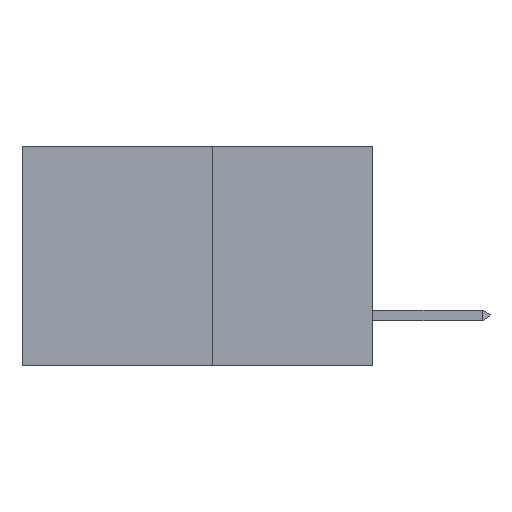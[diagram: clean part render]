
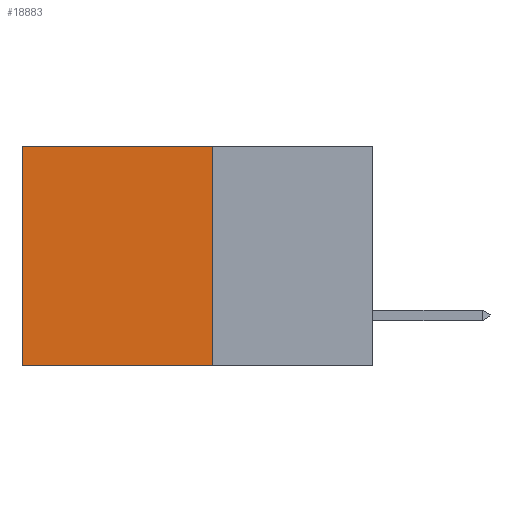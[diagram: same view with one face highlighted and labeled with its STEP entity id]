
A CAD part, left-side view. The second image highlights one B-rep face of the part: STEP entity #18883.
In plain terms, the highlighted planar face has unit normal (-1, 0, 0).
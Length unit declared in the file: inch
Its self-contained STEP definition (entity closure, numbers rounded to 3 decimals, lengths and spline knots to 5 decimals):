
#272 = LINE ( 'NONE', #681, #4980 ) ;
#427 = EDGE_CURVE ( 'NONE', #2098, #13107, #19022, .T. ) ;
#681 = CARTESIAN_POINT ( 'NONE',  ( 0.277, 0.27, -0.37 ) ) ;
#1015 = EDGE_CURVE ( 'NONE', #2098, #16600, #272, .T. ) ;
#1084 = VERTEX_POINT ( 'NONE', #19556 ) ;
#1745 = ORIENTED_EDGE ( 'NONE', *, *, #427, .T. ) ;
#1899 = CARTESIAN_POINT ( 'NONE',  ( 0.277, 0.27, 0. ) ) ;
#1974 = PLANE ( 'NONE',  #19280 ) ;
#2070 = DIRECTION ( 'NONE',  ( 1., 0., 0. ) ) ;
#2098 = VERTEX_POINT ( 'NONE', #1899 ) ;
#4743 = CARTESIAN_POINT ( 'NONE',  ( 0.277, 0.59, -0.37 ) ) ;
#4980 = VECTOR ( 'NONE', #21297, 39.37008 ) ;
#5964 = VECTOR ( 'NONE', #14572, 39.37008 ) ;
#6380 = CARTESIAN_POINT ( 'NONE',  ( 0.277, 0.27, -0.37 ) ) ;
#6897 = CARTESIAN_POINT ( 'NONE',  ( 0.277, 0.27, -0.37 ) ) ;
#6919 = DIRECTION ( 'NONE',  ( 0., 1., 0. ) ) ;
#7645 = LINE ( 'NONE', #6897, #13396 ) ;
#7882 = EDGE_CURVE ( 'NONE', #16600, #1084, #7645, .T. ) ;
#8899 = ORIENTED_EDGE ( 'NONE', *, *, #1015, .F. ) ;
#11194 = LINE ( 'NONE', #4743, #5964 ) ;
#11856 = EDGE_LOOP ( 'NONE', ( #18577, #19466, #8899, #1745 ) ) ;
#12308 = CARTESIAN_POINT ( 'NONE',  ( 0.277, 0.27, 0. ) ) ;
#13107 = VERTEX_POINT ( 'NONE', #17958 ) ;
#13396 = VECTOR ( 'NONE', #6919, 39.37008 ) ;
#13829 = CARTESIAN_POINT ( 'NONE',  ( 0.277, 0.27, -0.37 ) ) ;
#14572 = DIRECTION ( 'NONE',  ( 0., 0., -1. ) ) ;
#15781 = DIRECTION ( 'NONE',  ( 0., 0., -1. ) ) ;
#16600 = VERTEX_POINT ( 'NONE', #6380 ) ;
#16895 = FACE_OUTER_BOUND ( 'NONE', #11856, .T. ) ;
#17958 = CARTESIAN_POINT ( 'NONE',  ( 0.277, 0.59, 0. ) ) ;
#18051 = EDGE_CURVE ( 'NONE', #13107, #1084, #11194, .T. ) ;
#18409 = VECTOR ( 'NONE', #22072, 39.37008 ) ;
#18577 = ORIENTED_EDGE ( 'NONE', *, *, #18051, .T. ) ;
#18883 = ADVANCED_FACE ( 'NONE', ( #16895 ), #1974, .F. ) ;
#19022 = LINE ( 'NONE', #12308, #18409 ) ;
#19280 = AXIS2_PLACEMENT_3D ( 'NONE', #13829, #2070, #15781 ) ;
#19466 = ORIENTED_EDGE ( 'NONE', *, *, #7882, .F. ) ;
#19556 = CARTESIAN_POINT ( 'NONE',  ( 0.277, 0.59, -0.37 ) ) ;
#21297 = DIRECTION ( 'NONE',  ( 0., 0., -1. ) ) ;
#22072 = DIRECTION ( 'NONE',  ( 0., 1., 0. ) ) ;
